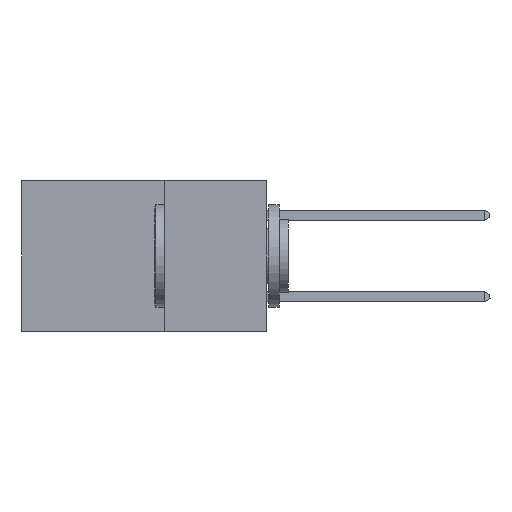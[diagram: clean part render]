
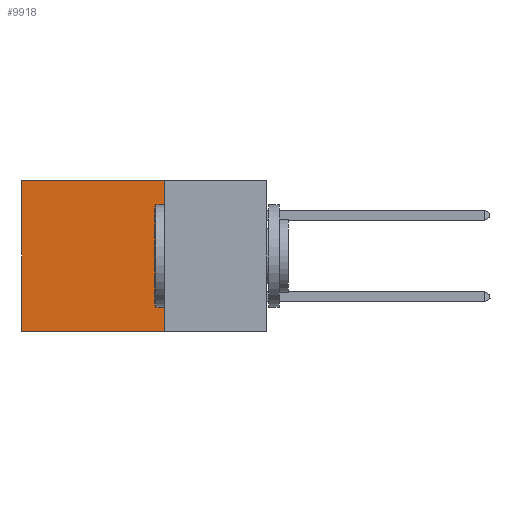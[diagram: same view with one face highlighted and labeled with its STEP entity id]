
A CAD part, left-side view. The second image highlights one B-rep face of the part: STEP entity #9918.
In plain terms, the highlighted planar face has unit normal (-1, 0, 0).
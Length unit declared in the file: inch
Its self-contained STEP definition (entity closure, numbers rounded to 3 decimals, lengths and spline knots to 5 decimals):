
#877 = VECTOR ( 'NONE', #23484, 39.37008 ) ;
#1885 = LINE ( 'NONE', #33097, #877 ) ;
#3751 = VECTOR ( 'NONE', #24836, 39.37008 ) ;
#4368 = ORIENTED_EDGE ( 'NONE', *, *, #27213, .T. ) ;
#5919 = DIRECTION ( 'NONE',  ( 0., 1., 0. ) ) ;
#6487 = DIRECTION ( 'NONE',  ( 1., 0., 0. ) ) ;
#6548 = EDGE_CURVE ( 'NONE', #22511, #30321, #40821, .T. ) ;
#8756 = LINE ( 'NONE', #21475, #3751 ) ;
#9918 = ADVANCED_FACE ( 'NONE', ( #34061 ), #13212, .F. ) ;
#13067 = CARTESIAN_POINT ( 'NONE',  ( 0.2875, 0.25, 0. ) ) ;
#13212 = PLANE ( 'NONE',  #35560 ) ;
#13580 = VECTOR ( 'NONE', #16587, 39.37008 ) ;
#14076 = VERTEX_POINT ( 'NONE', #14663 ) ;
#14663 = CARTESIAN_POINT ( 'NONE',  ( 0.2875, 0.25, 0. ) ) ;
#14867 = EDGE_CURVE ( 'NONE', #14076, #22511, #8756, .T. ) ;
#15575 = LINE ( 'NONE', #13067, #13580 ) ;
#16587 = DIRECTION ( 'NONE',  ( 0., 1., 0. ) ) ;
#16706 = EDGE_LOOP ( 'NONE', ( #4368, #39728, #23392, #36884 ) ) ;
#21475 = CARTESIAN_POINT ( 'NONE',  ( 0.2875, 0.25, 0. ) ) ;
#22233 = VECTOR ( 'NONE', #5919, 39.37008 ) ;
#22511 = VERTEX_POINT ( 'NONE', #26423 ) ;
#23392 = ORIENTED_EDGE ( 'NONE', *, *, #14867, .F. ) ;
#23431 = CARTESIAN_POINT ( 'NONE',  ( 0.2875, 0.6, -0.37 ) ) ;
#23484 = DIRECTION ( 'NONE',  ( 0., 0., -1. ) ) ;
#24810 = VERTEX_POINT ( 'NONE', #35143 ) ;
#24836 = DIRECTION ( 'NONE',  ( 0., 0., -1. ) ) ;
#25823 = CARTESIAN_POINT ( 'NONE',  ( 0.2875, 0.25, 0. ) ) ;
#26423 = CARTESIAN_POINT ( 'NONE',  ( 0.2875, 0.25, -0.37 ) ) ;
#27213 = EDGE_CURVE ( 'NONE', #24810, #30321, #1885, .T. ) ;
#28880 = DIRECTION ( 'NONE',  ( 0., 0., -1. ) ) ;
#30321 = VERTEX_POINT ( 'NONE', #23431 ) ;
#33097 = CARTESIAN_POINT ( 'NONE',  ( 0.2875, 0.6, 0. ) ) ;
#34061 = FACE_OUTER_BOUND ( 'NONE', #16706, .T. ) ;
#34626 = CARTESIAN_POINT ( 'NONE',  ( 0.2875, 0.25, -0.37 ) ) ;
#35143 = CARTESIAN_POINT ( 'NONE',  ( 0.2875, 0.6, 0. ) ) ;
#35560 = AXIS2_PLACEMENT_3D ( 'NONE', #25823, #6487, #28880 ) ;
#36662 = EDGE_CURVE ( 'NONE', #14076, #24810, #15575, .T. ) ;
#36884 = ORIENTED_EDGE ( 'NONE', *, *, #36662, .T. ) ;
#39728 = ORIENTED_EDGE ( 'NONE', *, *, #6548, .F. ) ;
#40821 = LINE ( 'NONE', #34626, #22233 ) ;
